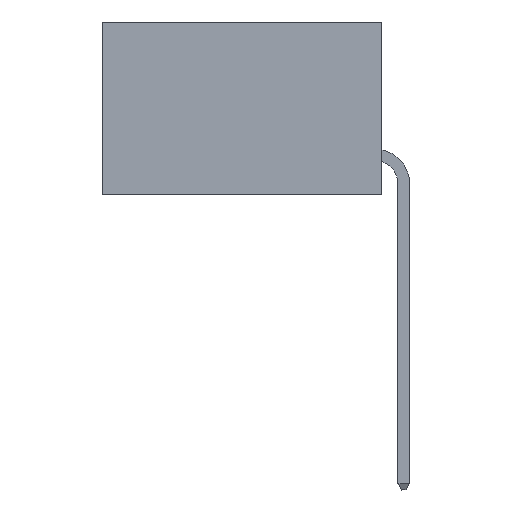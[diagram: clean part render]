
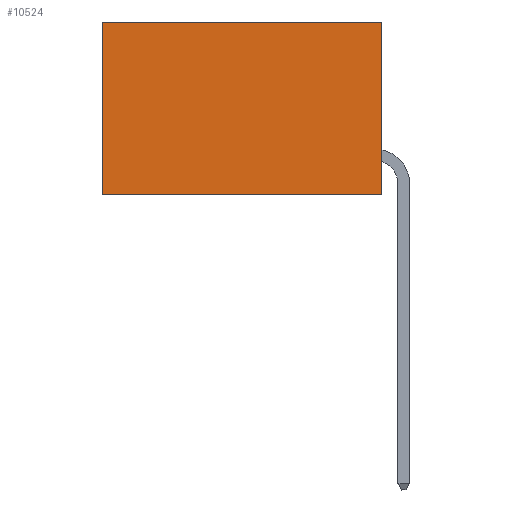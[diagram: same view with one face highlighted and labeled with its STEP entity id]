
A CAD part, left-side view. The second image highlights one B-rep face of the part: STEP entity #10524.
In plain terms, the highlighted planar face has unit normal (-1, 0, 0).
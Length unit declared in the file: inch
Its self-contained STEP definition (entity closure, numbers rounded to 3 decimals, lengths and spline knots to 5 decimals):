
#625 = DIRECTION ( 'NONE',  ( 0., 0., -1. ) ) ;
#1156 = VECTOR ( 'NONE', #625, 39.37008 ) ;
#1640 = EDGE_CURVE ( 'NONE', #21106, #16489, #29395, .T. ) ;
#2262 = ORIENTED_EDGE ( 'NONE', *, *, #2922, .T. ) ;
#2606 = CARTESIAN_POINT ( 'NONE',  ( 0.2875, 0., 0. ) ) ;
#2922 = EDGE_CURVE ( 'NONE', #24367, #16489, #9002, .T. ) ;
#2982 = DIRECTION ( 'NONE',  ( 1., 0., 0. ) ) ;
#3087 = PLANE ( 'NONE',  #21876 ) ;
#4261 = EDGE_LOOP ( 'NONE', ( #2262, #14819, #24343, #10481 ) ) ;
#5774 = CARTESIAN_POINT ( 'NONE',  ( 0.2875, 0., 0. ) ) ;
#5875 = DIRECTION ( 'NONE',  ( 0., 1., 0. ) ) ;
#6543 = CARTESIAN_POINT ( 'NONE',  ( 0.2875, 0.6, 0. ) ) ;
#6951 = VECTOR ( 'NONE', #17570, 39.37008 ) ;
#7662 = LINE ( 'NONE', #2606, #1156 ) ;
#9002 = LINE ( 'NONE', #15442, #13280 ) ;
#9799 = DIRECTION ( 'NONE',  ( 0., 0., -1. ) ) ;
#10481 = ORIENTED_EDGE ( 'NONE', *, *, #23511, .T. ) ;
#10524 = ADVANCED_FACE ( 'NONE', ( #12641 ), #3087, .F. ) ;
#10708 = CARTESIAN_POINT ( 'NONE',  ( 0.2875, 0., -0.37 ) ) ;
#12356 = CARTESIAN_POINT ( 'NONE',  ( 0.2875, 0., 0. ) ) ;
#12641 = FACE_OUTER_BOUND ( 'NONE', #4261, .T. ) ;
#12797 = VECTOR ( 'NONE', #5875, 39.37008 ) ;
#13280 = VECTOR ( 'NONE', #15535, 39.37008 ) ;
#14088 = EDGE_CURVE ( 'NONE', #25665, #21106, #7662, .T. ) ;
#14819 = ORIENTED_EDGE ( 'NONE', *, *, #1640, .F. ) ;
#15442 = CARTESIAN_POINT ( 'NONE',  ( 0.2875, 0.6, 0. ) ) ;
#15535 = DIRECTION ( 'NONE',  ( 0., 0., -1. ) ) ;
#16489 = VERTEX_POINT ( 'NONE', #21539 ) ;
#17570 = DIRECTION ( 'NONE',  ( 0., 1., 0. ) ) ;
#18978 = CARTESIAN_POINT ( 'NONE',  ( 0.2875, 0., 0. ) ) ;
#21106 = VERTEX_POINT ( 'NONE', #27261 ) ;
#21539 = CARTESIAN_POINT ( 'NONE',  ( 0.2875, 0.6, -0.37 ) ) ;
#21876 = AXIS2_PLACEMENT_3D ( 'NONE', #12356, #2982, #9799 ) ;
#22767 = LINE ( 'NONE', #5774, #12797 ) ;
#23511 = EDGE_CURVE ( 'NONE', #25665, #24367, #22767, .T. ) ;
#24343 = ORIENTED_EDGE ( 'NONE', *, *, #14088, .F. ) ;
#24367 = VERTEX_POINT ( 'NONE', #6543 ) ;
#25665 = VERTEX_POINT ( 'NONE', #18978 ) ;
#27261 = CARTESIAN_POINT ( 'NONE',  ( 0.2875, 0., -0.37 ) ) ;
#29395 = LINE ( 'NONE', #10708, #6951 ) ;
